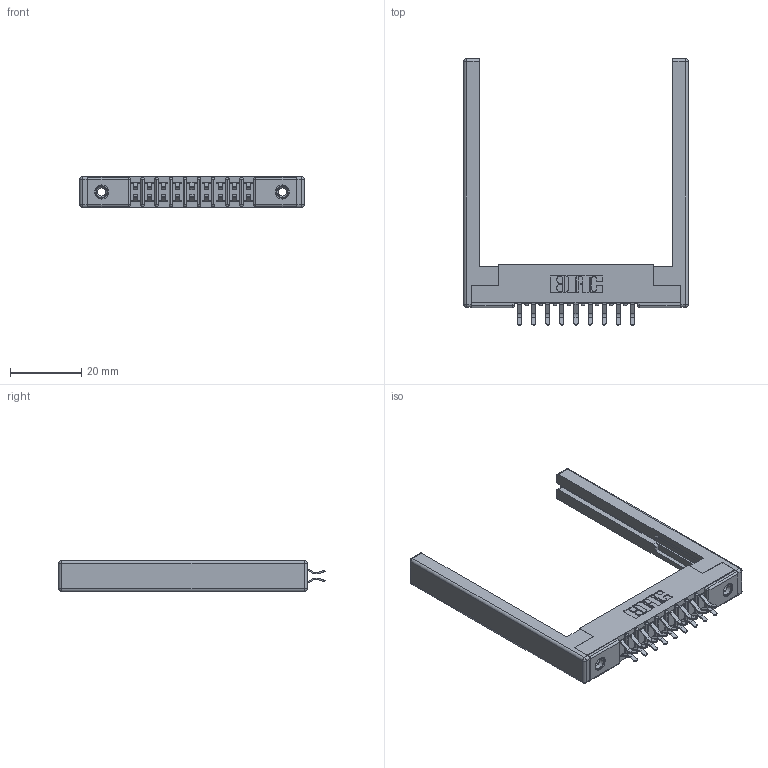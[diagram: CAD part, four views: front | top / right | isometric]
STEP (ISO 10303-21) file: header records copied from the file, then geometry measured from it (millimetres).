
FILE_DESCRIPTION (( 'STEP AP203' ), '1' );
FILE_NAME ('307-018-556-268.STEP', '2019-09-05T20:10:13', ( '' ), ( '' ), 'SwSTEP 2.0', 'SolidWorks 2016', '' );
FILE_SCHEMA (( 'CONFIG_CONTROL_DESIGN' ));
Length unit declared in the file: inch
Products named in the file (5): 307-290-001_556; 345-250-001_345-250-001-102; 307-220-068; 307-018-556-268; 307 Part_.156 Dia Mounting Holes
Assembly tree (23 placements, depth 2):
  307-018-556-268
    307 Part_.156 Dia Mounting Holes
    307-290-001_556  x18
    307-220-068  x2
    345-250-001_345-250-001-102  x2
Bounding box: 63.09 x 74.93 x 8.71 mm (x, y, z)
Volume: 8686.7 mm3; surface area: 10634.1 mm2
Topology: 23 solids, 23 shells, 1182 faces, 3269 edges, 2106 vertices
Faces by surface type: plane 752, cylinder 386, sphere 28, cone 12, torus 4
Entity records: 14935 total; most frequent: CARTESIAN_POINT 2430, DIRECTION 2410, ORIENTED_EDGE 2396, EDGE_CURVE 1198, VECTOR 902, LINE 902, VERTEX_POINT 774, AXIS2_PLACEMENT_3D 754
